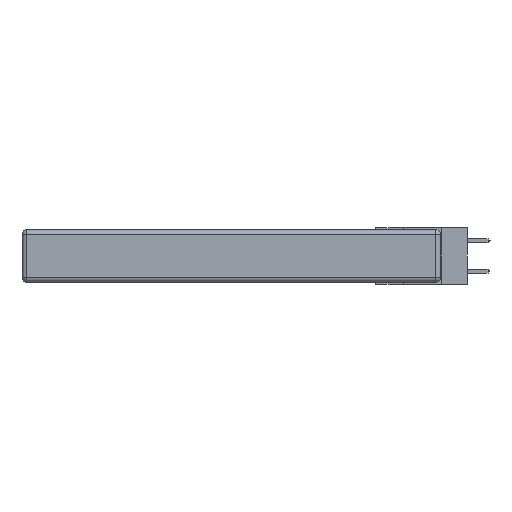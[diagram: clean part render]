
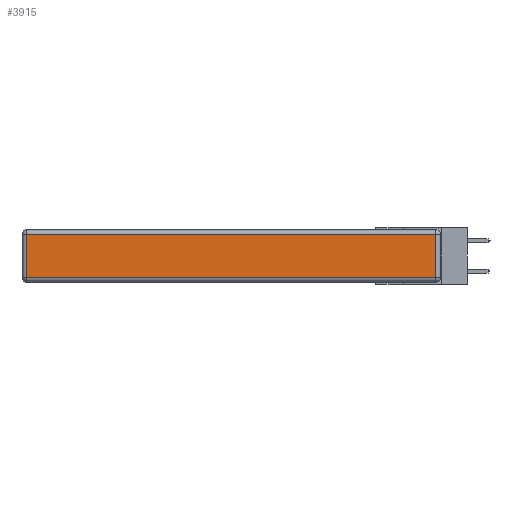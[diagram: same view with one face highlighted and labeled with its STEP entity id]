
A CAD part, left-side view. The second image highlights one B-rep face of the part: STEP entity #3915.
In plain terms, the highlighted planar face has unit normal (-1, 0, 0).
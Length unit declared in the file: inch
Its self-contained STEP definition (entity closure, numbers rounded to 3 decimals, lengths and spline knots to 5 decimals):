
#21 = DIRECTION ( 'NONE',  ( 0., 0., 1. ) ) ;
#321 = VERTEX_POINT ( 'NONE', #8764 ) ;
#917 = VECTOR ( 'NONE', #3700, 39.37008 ) ;
#1438 = VERTEX_POINT ( 'NONE', #9292 ) ;
#1524 = EDGE_CURVE ( 'NONE', #2318, #1438, #3118, .T. ) ;
#2071 = VECTOR ( 'NONE', #10539, 39.37008 ) ;
#2318 = VERTEX_POINT ( 'NONE', #11288 ) ;
#2766 = FACE_OUTER_BOUND ( 'NONE', #6128, .T. ) ;
#3118 = LINE ( 'NONE', #10309, #6579 ) ;
#3196 = ORIENTED_EDGE ( 'NONE', *, *, #4079, .T. ) ;
#3700 = DIRECTION ( 'NONE',  ( 0., 0., -1. ) ) ;
#3915 = ADVANCED_FACE ( 'NONE', ( #2766 ), #10937, .T. ) ;
#4079 = EDGE_CURVE ( 'NONE', #10443, #2318, #8307, .T. ) ;
#4116 = CARTESIAN_POINT ( 'NONE',  ( 0., 0.03, -0.343 ) ) ;
#4662 = LINE ( 'NONE', #7371, #2071 ) ;
#4805 = CARTESIAN_POINT ( 'NONE',  ( 0., 2.72, -0.343 ) ) ;
#4971 = EDGE_CURVE ( 'NONE', #321, #10443, #4662, .T. ) ;
#5309 = ORIENTED_EDGE ( 'NONE', *, *, #12219, .T. ) ;
#5763 = DIRECTION ( 'NONE',  ( -1., 0., 0. ) ) ;
#5885 = CARTESIAN_POINT ( 'NONE',  ( 0., 0.03, -0.313 ) ) ;
#5948 = DIRECTION ( 'NONE',  ( 0., 1., 0. ) ) ;
#6128 = EDGE_LOOP ( 'NONE', ( #11160, #3196, #8110, #5309 ) ) ;
#6579 = VECTOR ( 'NONE', #5948, 39.37008 ) ;
#7371 = CARTESIAN_POINT ( 'NONE',  ( 0., 0., -0.313 ) ) ;
#8110 = ORIENTED_EDGE ( 'NONE', *, *, #1524, .T. ) ;
#8307 = LINE ( 'NONE', #4116, #9963 ) ;
#8764 = CARTESIAN_POINT ( 'NONE',  ( 0., 2.72, -0.313 ) ) ;
#8933 = AXIS2_PLACEMENT_3D ( 'NONE', #10061, #5763, #9970 ) ;
#9292 = CARTESIAN_POINT ( 'NONE',  ( 0., 2.72, -0.03 ) ) ;
#9691 = LINE ( 'NONE', #4805, #917 ) ;
#9963 = VECTOR ( 'NONE', #21, 39.37008 ) ;
#9970 = DIRECTION ( 'NONE',  ( 0., 0., 1. ) ) ;
#10061 = CARTESIAN_POINT ( 'NONE',  ( 0., 0., -0.343 ) ) ;
#10309 = CARTESIAN_POINT ( 'NONE',  ( 0., 2.75, -0.03 ) ) ;
#10443 = VERTEX_POINT ( 'NONE', #5885 ) ;
#10539 = DIRECTION ( 'NONE',  ( 0., -1., 0. ) ) ;
#10937 = PLANE ( 'NONE',  #8933 ) ;
#11160 = ORIENTED_EDGE ( 'NONE', *, *, #4971, .T. ) ;
#11288 = CARTESIAN_POINT ( 'NONE',  ( 0., 0.03, -0.03 ) ) ;
#12219 = EDGE_CURVE ( 'NONE', #1438, #321, #9691, .T. ) ;
